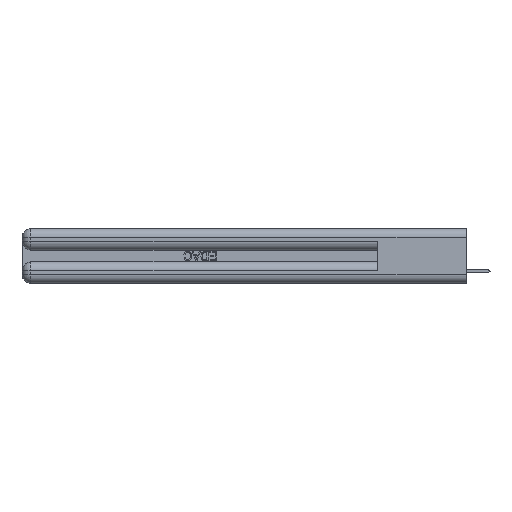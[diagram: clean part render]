
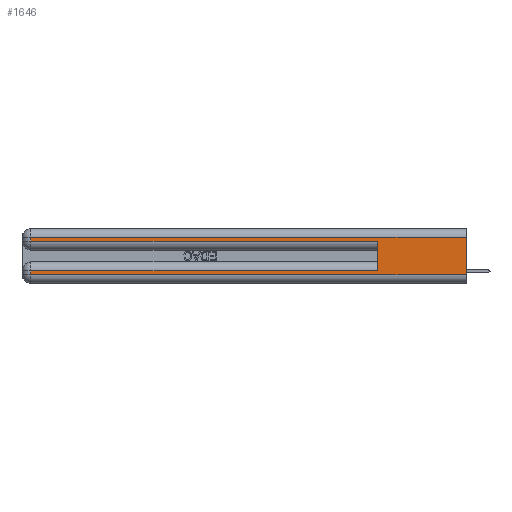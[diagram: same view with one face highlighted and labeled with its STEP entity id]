
A CAD part, left-side view. The second image highlights one B-rep face of the part: STEP entity #1646.
In plain terms, the highlighted planar face has unit normal (-1, 0, 0).
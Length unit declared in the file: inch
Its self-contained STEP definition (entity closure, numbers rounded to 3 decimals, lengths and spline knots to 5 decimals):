
#416 = PLANE ( 'NONE',  #3846 ) ;
#697 = VECTOR ( 'NONE', #35525, 39.37008 ) ;
#1646 = ADVANCED_FACE ( 'NONE', ( #44706 ), #416, .F. ) ;
#2621 = LINE ( 'NONE', #50437, #51962 ) ;
#2997 = VECTOR ( 'NONE', #9335, 39.37008 ) ;
#3485 = DIRECTION ( 'NONE',  ( 0., 0., -1. ) ) ;
#3698 = CARTESIAN_POINT ( 'NONE',  ( 0., 2.94, 0.31 ) ) ;
#3846 = AXIS2_PLACEMENT_3D ( 'NONE', #46636, #23591, #3485 ) ;
#5409 = CARTESIAN_POINT ( 'NONE',  ( 0., 0., 0.31 ) ) ;
#5835 = EDGE_CURVE ( 'NONE', #26192, #6686, #25981, .T. ) ;
#6626 = VECTOR ( 'NONE', #26668, 39.37008 ) ;
#6686 = VERTEX_POINT ( 'NONE', #34619 ) ;
#7010 = CARTESIAN_POINT ( 'NONE',  ( 0., 0., 0.31 ) ) ;
#7198 = ORIENTED_EDGE ( 'NONE', *, *, #17853, .T. ) ;
#9335 = DIRECTION ( 'NONE',  ( 0., 0., -1. ) ) ;
#13309 = EDGE_CURVE ( 'NONE', #6686, #39734, #24809, .T. ) ;
#14419 = VECTOR ( 'NONE', #43966, 39.37008 ) ;
#15064 = CARTESIAN_POINT ( 'NONE',  ( 0., 0.6, 0.145 ) ) ;
#15457 = CARTESIAN_POINT ( 'NONE',  ( 0., 2.94, 0.285 ) ) ;
#16240 = EDGE_CURVE ( 'NONE', #21457, #24987, #2621, .T. ) ;
#17853 = EDGE_CURVE ( 'NONE', #24987, #48564, #32177, .T. ) ;
#17964 = CARTESIAN_POINT ( 'NONE',  ( 0., 2.94, 0.06 ) ) ;
#18947 = VECTOR ( 'NONE', #50363, 39.37008 ) ;
#19508 = EDGE_CURVE ( 'NONE', #52136, #33589, #20625, .T. ) ;
#20581 = ORIENTED_EDGE ( 'NONE', *, *, #16240, .T. ) ;
#20625 = LINE ( 'NONE', #23553, #2997 ) ;
#21457 = VERTEX_POINT ( 'NONE', #3698 ) ;
#22106 = EDGE_CURVE ( 'NONE', #52136, #21457, #34634, .T. ) ;
#23553 = CARTESIAN_POINT ( 'NONE',  ( 0., 0., 0.37 ) ) ;
#23591 = DIRECTION ( 'NONE',  ( 1., 0., 0. ) ) ;
#23979 = EDGE_CURVE ( 'NONE', #26192, #48564, #31963, .T. ) ;
#24325 = CARTESIAN_POINT ( 'NONE',  ( 0., 0.6, 0.285 ) ) ;
#24683 = EDGE_LOOP ( 'NONE', ( #38156, #47936, #20581, #7198, #29648, #28673, #48392, #47428 ) ) ;
#24809 = LINE ( 'NONE', #30645, #49428 ) ;
#24987 = VERTEX_POINT ( 'NONE', #15457 ) ;
#25981 = LINE ( 'NONE', #51144, #697 ) ;
#26192 = VERTEX_POINT ( 'NONE', #42118 ) ;
#26668 = DIRECTION ( 'NONE',  ( 0., 0., 1. ) ) ;
#26735 = DIRECTION ( 'NONE',  ( 0., 0., -1. ) ) ;
#28673 = ORIENTED_EDGE ( 'NONE', *, *, #5835, .T. ) ;
#29648 = ORIENTED_EDGE ( 'NONE', *, *, #23979, .F. ) ;
#29655 = LINE ( 'NONE', #50162, #18947 ) ;
#30645 = CARTESIAN_POINT ( 'NONE',  ( 0., 2.94, 0.37 ) ) ;
#31963 = LINE ( 'NONE', #15064, #6626 ) ;
#32177 = LINE ( 'NONE', #48550, #14419 ) ;
#32263 = DIRECTION ( 'NONE',  ( 0., 0., -1. ) ) ;
#33589 = VERTEX_POINT ( 'NONE', #42724 ) ;
#34619 = CARTESIAN_POINT ( 'NONE',  ( 0., 2.94, 0.085 ) ) ;
#34634 = LINE ( 'NONE', #5409, #40945 ) ;
#35525 = DIRECTION ( 'NONE',  ( 0., 1., 0. ) ) ;
#38156 = ORIENTED_EDGE ( 'NONE', *, *, #19508, .F. ) ;
#39734 = VERTEX_POINT ( 'NONE', #17964 ) ;
#40945 = VECTOR ( 'NONE', #42465, 39.37008 ) ;
#42118 = CARTESIAN_POINT ( 'NONE',  ( 0., 0.6, 0.085 ) ) ;
#42465 = DIRECTION ( 'NONE',  ( 0., 1., 0. ) ) ;
#42724 = CARTESIAN_POINT ( 'NONE',  ( 0., 0., 0.06 ) ) ;
#43966 = DIRECTION ( 'NONE',  ( 0., -1., 0. ) ) ;
#44706 = FACE_OUTER_BOUND ( 'NONE', #24683, .T. ) ;
#46636 = CARTESIAN_POINT ( 'NONE',  ( 0., 0., 0.37 ) ) ;
#47428 = ORIENTED_EDGE ( 'NONE', *, *, #48819, .T. ) ;
#47936 = ORIENTED_EDGE ( 'NONE', *, *, #22106, .T. ) ;
#48392 = ORIENTED_EDGE ( 'NONE', *, *, #13309, .T. ) ;
#48550 = CARTESIAN_POINT ( 'NONE',  ( 0., 0., 0.285 ) ) ;
#48564 = VERTEX_POINT ( 'NONE', #24325 ) ;
#48819 = EDGE_CURVE ( 'NONE', #39734, #33589, #29655, .T. ) ;
#49428 = VECTOR ( 'NONE', #26735, 39.37008 ) ;
#50162 = CARTESIAN_POINT ( 'NONE',  ( 0., 0., 0.06 ) ) ;
#50363 = DIRECTION ( 'NONE',  ( 0., -1., 0. ) ) ;
#50437 = CARTESIAN_POINT ( 'NONE',  ( 0., 2.94, 0.37 ) ) ;
#51144 = CARTESIAN_POINT ( 'NONE',  ( 0., 0., 0.085 ) ) ;
#51962 = VECTOR ( 'NONE', #32263, 39.37008 ) ;
#52136 = VERTEX_POINT ( 'NONE', #7010 ) ;
